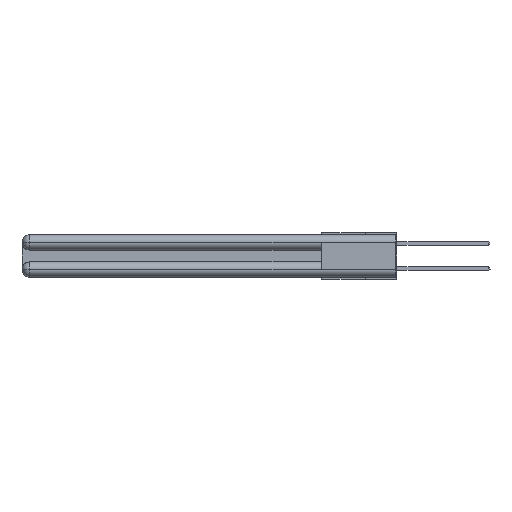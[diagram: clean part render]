
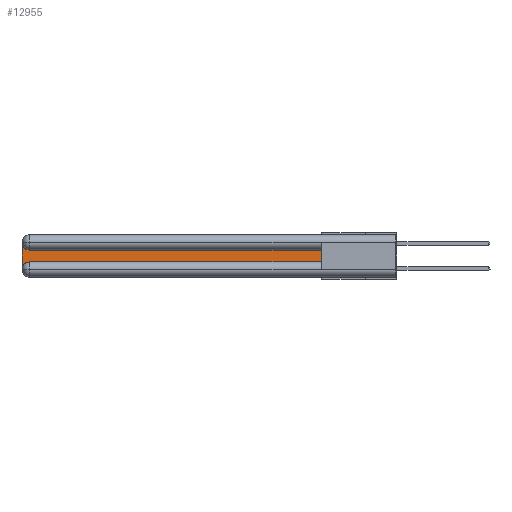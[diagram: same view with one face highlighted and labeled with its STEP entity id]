
A CAD part, left-side view. The second image highlights one B-rep face of the part: STEP entity #12955.
In plain terms, the highlighted planar face has unit normal (-1, 0, 0).
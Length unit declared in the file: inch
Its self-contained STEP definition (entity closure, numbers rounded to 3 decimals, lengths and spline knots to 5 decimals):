
#843 = CARTESIAN_POINT ( 'NONE',  ( 0.075, 3., -0.1225 ) ) ;
#958 = DIRECTION ( 'NONE',  ( 0., 0., -1. ) ) ;
#1142 = EDGE_CURVE ( 'NONE', #23552, #7404, #11185, .T. ) ;
#1229 = DIRECTION ( 'NONE',  ( 0., -1., 0. ) ) ;
#1798 = CARTESIAN_POINT ( 'NONE',  ( 0.075, 0.6, -0.1225 ) ) ;
#2825 = ORIENTED_EDGE ( 'NONE', *, *, #27053, .T. ) ;
#3901 = ORIENTED_EDGE ( 'NONE', *, *, #24781, .T. ) ;
#4975 = CIRCLE ( 'NONE', #30389, 0.06 ) ;
#5584 = DIRECTION ( 'NONE',  ( 0., 0., -1. ) ) ;
#5887 = EDGE_CURVE ( 'NONE', #7404, #19330, #29050, .T. ) ;
#7404 = VERTEX_POINT ( 'NONE', #26037 ) ;
#8408 = VECTOR ( 'NONE', #11504, 39.37008 ) ;
#9301 = VERTEX_POINT ( 'NONE', #23380 ) ;
#10294 = LINE ( 'NONE', #11263, #31545 ) ;
#11185 = LINE ( 'NONE', #19258, #28916 ) ;
#11263 = CARTESIAN_POINT ( 'NONE',  ( 0.075, 0.6, -0.2175 ) ) ;
#11294 = LINE ( 'NONE', #1798, #15590 ) ;
#11504 = DIRECTION ( 'NONE',  ( 0., 0., 1. ) ) ;
#12146 = CARTESIAN_POINT ( 'NONE',  ( 0.075, 2.94, -0.2175 ) ) ;
#12955 = ADVANCED_FACE ( 'NONE', ( #24109 ), #16033, .F. ) ;
#14618 = CARTESIAN_POINT ( 'NONE',  ( 0.075, 0.6, -0.2175 ) ) ;
#14933 = CARTESIAN_POINT ( 'NONE',  ( 0.075, 0.6, -0.1225 ) ) ;
#15506 = DIRECTION ( 'NONE',  ( 0., 0., -1. ) ) ;
#15590 = VECTOR ( 'NONE', #24696, 39.37008 ) ;
#16033 = PLANE ( 'NONE',  #25485 ) ;
#17905 = CARTESIAN_POINT ( 'NONE',  ( 0.075, 2.94, -0.0625 ) ) ;
#18129 = DIRECTION ( 'NONE',  ( 1., 0., 0. ) ) ;
#18442 = DIRECTION ( 'NONE',  ( 1., 0., 0. ) ) ;
#19146 = EDGE_CURVE ( 'NONE', #20000, #25836, #28127, .T. ) ;
#19258 = CARTESIAN_POINT ( 'NONE',  ( 0.075, 3., -0.2175 ) ) ;
#19330 = VERTEX_POINT ( 'NONE', #12146 ) ;
#19865 = ORIENTED_EDGE ( 'NONE', *, *, #19146, .T. ) ;
#20000 = VERTEX_POINT ( 'NONE', #14618 ) ;
#22764 = ORIENTED_EDGE ( 'NONE', *, *, #1142, .T. ) ;
#23380 = CARTESIAN_POINT ( 'NONE',  ( 0.075, 2.94, -0.1225 ) ) ;
#23552 = VERTEX_POINT ( 'NONE', #24605 ) ;
#24109 = FACE_OUTER_BOUND ( 'NONE', #31338, .T. ) ;
#24347 = DIRECTION ( 'NONE',  ( 0., 0., -1. ) ) ;
#24472 = ORIENTED_EDGE ( 'NONE', *, *, #5887, .T. ) ;
#24605 = CARTESIAN_POINT ( 'NONE',  ( 0.075, 3., -0.0625 ) ) ;
#24696 = DIRECTION ( 'NONE',  ( 0., 1., 0. ) ) ;
#24781 = EDGE_CURVE ( 'NONE', #19330, #20000, #10294, .T. ) ;
#25420 = ORIENTED_EDGE ( 'NONE', *, *, #29565, .T. ) ;
#25485 = AXIS2_PLACEMENT_3D ( 'NONE', #843, #18442, #958 ) ;
#25836 = VERTEX_POINT ( 'NONE', #14933 ) ;
#26037 = CARTESIAN_POINT ( 'NONE',  ( 0.075, 3., -0.2775 ) ) ;
#26705 = CARTESIAN_POINT ( 'NONE',  ( 0.075, 0.6, -0.2175 ) ) ;
#27053 = EDGE_CURVE ( 'NONE', #9301, #23552, #4975, .T. ) ;
#27955 = DIRECTION ( 'NONE',  ( 1., 0., 0. ) ) ;
#28127 = LINE ( 'NONE', #26705, #8408 ) ;
#28916 = VECTOR ( 'NONE', #24347, 39.37008 ) ;
#29050 = CIRCLE ( 'NONE', #29418, 0.06 ) ;
#29418 = AXIS2_PLACEMENT_3D ( 'NONE', #32380, #27955, #5584 ) ;
#29565 = EDGE_CURVE ( 'NONE', #25836, #9301, #11294, .T. ) ;
#30389 = AXIS2_PLACEMENT_3D ( 'NONE', #17905, #18129, #15506 ) ;
#31338 = EDGE_LOOP ( 'NONE', ( #25420, #2825, #22764, #24472, #3901, #19865 ) ) ;
#31545 = VECTOR ( 'NONE', #1229, 39.37008 ) ;
#32380 = CARTESIAN_POINT ( 'NONE',  ( 0.075, 2.94, -0.2775 ) ) ;
